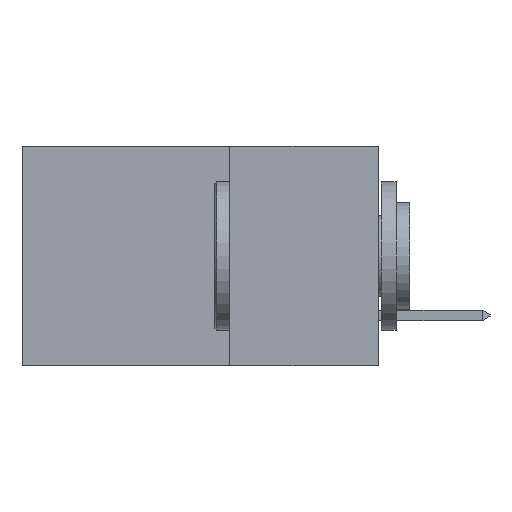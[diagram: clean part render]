
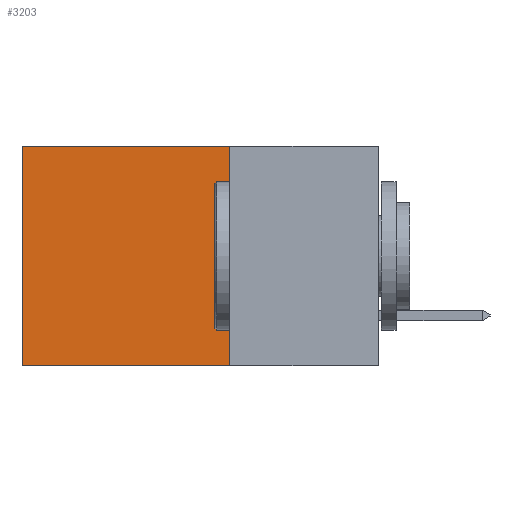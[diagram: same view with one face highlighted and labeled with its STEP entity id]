
A CAD part, left-side view. The second image highlights one B-rep face of the part: STEP entity #3203.
In plain terms, the highlighted planar face has unit normal (-1, 0, 0).
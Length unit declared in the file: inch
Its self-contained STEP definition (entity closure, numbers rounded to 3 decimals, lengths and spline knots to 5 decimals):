
#223 = VECTOR ( 'NONE', #19351, 39.37008 ) ;
#847 = ORIENTED_EDGE ( 'NONE', *, *, #10490, .T. ) ;
#1636 = PLANE ( 'NONE',  #14861 ) ;
#1667 = LINE ( 'NONE', #3889, #6713 ) ;
#3154 = CARTESIAN_POINT ( 'NONE',  ( 0.298, 0.25, -0.37 ) ) ;
#3203 = ADVANCED_FACE ( 'NONE', ( #7870 ), #1636, .F. ) ;
#3590 = EDGE_CURVE ( 'NONE', #10664, #14887, #20316, .T. ) ;
#3889 = CARTESIAN_POINT ( 'NONE',  ( 0.298, 0.25, -0.37 ) ) ;
#6622 = CARTESIAN_POINT ( 'NONE',  ( 0.298, 0.25, 0. ) ) ;
#6713 = VECTOR ( 'NONE', #18675, 39.37008 ) ;
#7870 = FACE_OUTER_BOUND ( 'NONE', #23540, .T. ) ;
#8174 = ORIENTED_EDGE ( 'NONE', *, *, #3590, .T. ) ;
#8514 = VECTOR ( 'NONE', #9862, 39.37008 ) ;
#8604 = EDGE_CURVE ( 'NONE', #21677, #14887, #1667, .T. ) ;
#9862 = DIRECTION ( 'NONE',  ( 0., 0., -1. ) ) ;
#10490 = EDGE_CURVE ( 'NONE', #17592, #10664, #21621, .T. ) ;
#10664 = VERTEX_POINT ( 'NONE', #15318 ) ;
#10855 = CARTESIAN_POINT ( 'NONE',  ( 0.298, 0.6, -0.37 ) ) ;
#11694 = LINE ( 'NONE', #6622, #223 ) ;
#11702 = ORIENTED_EDGE ( 'NONE', *, *, #24629, .F. ) ;
#14795 = DIRECTION ( 'NONE',  ( 0., 0., -1. ) ) ;
#14861 = AXIS2_PLACEMENT_3D ( 'NONE', #15114, #14889, #14795 ) ;
#14887 = VERTEX_POINT ( 'NONE', #10855 ) ;
#14889 = DIRECTION ( 'NONE',  ( 1., 0., 0. ) ) ;
#15009 = CARTESIAN_POINT ( 'NONE',  ( 0.298, 0.6, 0. ) ) ;
#15114 = CARTESIAN_POINT ( 'NONE',  ( 0.298, 0.25, 0. ) ) ;
#15318 = CARTESIAN_POINT ( 'NONE',  ( 0.298, 0.6, 0. ) ) ;
#16901 = DIRECTION ( 'NONE',  ( 0., 1., 0. ) ) ;
#17592 = VERTEX_POINT ( 'NONE', #20575 ) ;
#18675 = DIRECTION ( 'NONE',  ( 0., 1., 0. ) ) ;
#19351 = DIRECTION ( 'NONE',  ( 0., 0., -1. ) ) ;
#19868 = ORIENTED_EDGE ( 'NONE', *, *, #8604, .F. ) ;
#20316 = LINE ( 'NONE', #15009, #8514 ) ;
#20575 = CARTESIAN_POINT ( 'NONE',  ( 0.298, 0.25, 0. ) ) ;
#21621 = LINE ( 'NONE', #26977, #22255 ) ;
#21677 = VERTEX_POINT ( 'NONE', #3154 ) ;
#22255 = VECTOR ( 'NONE', #16901, 39.37008 ) ;
#23540 = EDGE_LOOP ( 'NONE', ( #8174, #19868, #11702, #847 ) ) ;
#24629 = EDGE_CURVE ( 'NONE', #17592, #21677, #11694, .T. ) ;
#26977 = CARTESIAN_POINT ( 'NONE',  ( 0.298, 0.25, 0. ) ) ;
